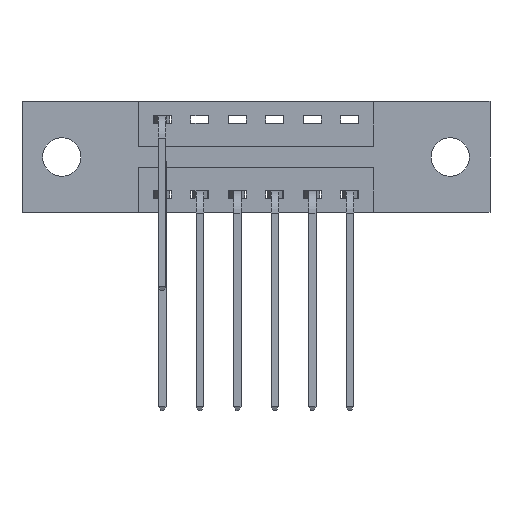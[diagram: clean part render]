
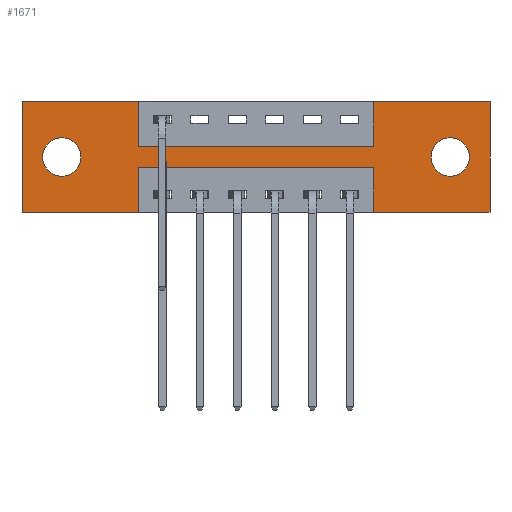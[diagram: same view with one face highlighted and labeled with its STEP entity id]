
A CAD part, front view. The second image highlights one B-rep face of the part: STEP entity #1671.
In plain terms, the highlighted planar face has unit normal (0, -1, 0).
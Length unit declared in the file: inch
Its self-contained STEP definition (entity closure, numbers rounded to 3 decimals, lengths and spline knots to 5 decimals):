
#90 = CARTESIAN_POINT ( 'NONE',  ( 0.3875, 0., -0.15 ) ) ;
#202 = DIRECTION ( 'NONE',  ( -1., 0., 0. ) ) ;
#394 = VERTEX_POINT ( 'NONE', #4883 ) ;
#474 = CARTESIAN_POINT ( 'NONE',  ( 0.3875, 0., 0. ) ) ;
#492 = CARTESIAN_POINT ( 'NONE',  ( 0.3875, 0., 0. ) ) ;
#529 = CARTESIAN_POINT ( 'NONE',  ( 0.3875, 0., -0.37 ) ) ;
#636 = EDGE_LOOP ( 'NONE', ( #1994, #3930 ) ) ;
#640 = DIRECTION ( 'NONE',  ( 0., 0., 1. ) ) ;
#740 = VERTEX_POINT ( 'NONE', #492 ) ;
#747 = DIRECTION ( 'NONE',  ( 0., 1., 0. ) ) ;
#805 = FACE_OUTER_BOUND ( 'NONE', #9752, .T. ) ;
#927 = DIRECTION ( 'NONE',  ( 1., 0., 0. ) ) ;
#945 = VECTOR ( 'NONE', #6337, 39.37008 ) ;
#1133 = DIRECTION ( 'NONE',  ( 0., 1., 0. ) ) ;
#1139 = VERTEX_POINT ( 'NONE', #9438 ) ;
#1234 = VECTOR ( 'NONE', #640, 39.37008 ) ;
#1249 = VERTEX_POINT ( 'NONE', #1520 ) ;
#1357 = FACE_BOUND ( 'NONE', #7469, .T. ) ;
#1470 = EDGE_CURVE ( 'NONE', #5039, #4502, #3247, .T. ) ;
#1492 = LINE ( 'NONE', #8779, #1234 ) ;
#1520 = CARTESIAN_POINT ( 'NONE',  ( 1.1725, 0., -0.15 ) ) ;
#1593 = ORIENTED_EDGE ( 'NONE', *, *, #6274, .F. ) ;
#1630 = AXIS2_PLACEMENT_3D ( 'NONE', #6113, #1133, #6923 ) ;
#1663 = VERTEX_POINT ( 'NONE', #4180 ) ;
#1671 = ADVANCED_FACE ( 'NONE', ( #3384, #1357, #805 ), #9903, .T. ) ;
#1941 = LINE ( 'NONE', #90, #3419 ) ;
#1994 = ORIENTED_EDGE ( 'NONE', *, *, #7190, .T. ) ;
#2124 = VERTEX_POINT ( 'NONE', #6294 ) ;
#2141 = DIRECTION ( 'NONE',  ( 1., 0., 0. ) ) ;
#2580 = LINE ( 'NONE', #8137, #9216 ) ;
#2625 = VECTOR ( 'NONE', #4668, 39.37008 ) ;
#2714 = EDGE_CURVE ( 'NONE', #3999, #8539, #7148, .T. ) ;
#2780 = AXIS2_PLACEMENT_3D ( 'NONE', #9144, #7848, #4446 ) ;
#2950 = CIRCLE ( 'NONE', #5992, 0.064 ) ;
#2985 = ORIENTED_EDGE ( 'NONE', *, *, #6640, .T. ) ;
#3200 = EDGE_CURVE ( 'NONE', #394, #6590, #8996, .T. ) ;
#3211 = ORIENTED_EDGE ( 'NONE', *, *, #8750, .F. ) ;
#3247 = LINE ( 'NONE', #10345, #9323 ) ;
#3329 = CARTESIAN_POINT ( 'NONE',  ( 1.4275, 0., -0.185 ) ) ;
#3384 = FACE_BOUND ( 'NONE', #636, .T. ) ;
#3402 = ORIENTED_EDGE ( 'NONE', *, *, #3988, .F. ) ;
#3419 = VECTOR ( 'NONE', #927, 39.37008 ) ;
#3431 = EDGE_CURVE ( 'NONE', #740, #1663, #4963, .T. ) ;
#3490 = ORIENTED_EDGE ( 'NONE', *, *, #9827, .T. ) ;
#3673 = CARTESIAN_POINT ( 'NONE',  ( 0., 0., 0. ) ) ;
#3804 = ORIENTED_EDGE ( 'NONE', *, *, #5069, .F. ) ;
#3930 = ORIENTED_EDGE ( 'NONE', *, *, #2714, .T. ) ;
#3988 = EDGE_CURVE ( 'NONE', #1663, #1249, #1941, .T. ) ;
#3999 = VERTEX_POINT ( 'NONE', #5901 ) ;
#4078 = CARTESIAN_POINT ( 'NONE',  ( 0., 0., 0. ) ) ;
#4165 = DIRECTION ( 'NONE',  ( 0., 0., -1. ) ) ;
#4180 = CARTESIAN_POINT ( 'NONE',  ( 0.3875, 0., -0.15 ) ) ;
#4211 = DIRECTION ( 'NONE',  ( 0., 0., 1. ) ) ;
#4364 = CIRCLE ( 'NONE', #9843, 0.064 ) ;
#4430 = CARTESIAN_POINT ( 'NONE',  ( 0., 0., -0.37 ) ) ;
#4446 = DIRECTION ( 'NONE',  ( 0., 0., -1. ) ) ;
#4502 = VERTEX_POINT ( 'NONE', #7299 ) ;
#4541 = EDGE_CURVE ( 'NONE', #1249, #7919, #2580, .T. ) ;
#4642 = DIRECTION ( 'NONE',  ( 0., -1., 0. ) ) ;
#4668 = DIRECTION ( 'NONE',  ( -1., 0., 0. ) ) ;
#4714 = DIRECTION ( 'NONE',  ( 0., 0., -1. ) ) ;
#4853 = VECTOR ( 'NONE', #6493, 39.37008 ) ;
#4883 = CARTESIAN_POINT ( 'NONE',  ( 0., 0., -0.37 ) ) ;
#4946 = CARTESIAN_POINT ( 'NONE',  ( 0., 0., -0.37 ) ) ;
#4963 = LINE ( 'NONE', #474, #6814 ) ;
#5039 = VERTEX_POINT ( 'NONE', #7229 ) ;
#5069 = EDGE_CURVE ( 'NONE', #10313, #1139, #1492, .T. ) ;
#5149 = ORIENTED_EDGE ( 'NONE', *, *, #1470, .F. ) ;
#5151 = LINE ( 'NONE', #10004, #7263 ) ;
#5500 = LINE ( 'NONE', #7042, #5964 ) ;
#5536 = ORIENTED_EDGE ( 'NONE', *, *, #8371, .F. ) ;
#5548 = CARTESIAN_POINT ( 'NONE',  ( 0.3875, 0., -0.22 ) ) ;
#5590 = EDGE_CURVE ( 'NONE', #1139, #8738, #9538, .T. ) ;
#5673 = CARTESIAN_POINT ( 'NONE',  ( 0.1325, 0., -0.121 ) ) ;
#5721 = CARTESIAN_POINT ( 'NONE',  ( 1.1725, 0., 0. ) ) ;
#5766 = CARTESIAN_POINT ( 'NONE',  ( 0.1325, 0., -0.185 ) ) ;
#5901 = CARTESIAN_POINT ( 'NONE',  ( 1.4275, 0., -0.249 ) ) ;
#5964 = VECTOR ( 'NONE', #2141, 39.37008 ) ;
#5985 = DIRECTION ( 'NONE',  ( 0., 0., -1. ) ) ;
#5990 = LINE ( 'NONE', #4078, #9882 ) ;
#5992 = AXIS2_PLACEMENT_3D ( 'NONE', #3329, #8870, #4165 ) ;
#6084 = ORIENTED_EDGE ( 'NONE', *, *, #3200, .F. ) ;
#6113 = CARTESIAN_POINT ( 'NONE',  ( 0.1325, 0., -0.185 ) ) ;
#6122 = EDGE_CURVE ( 'NONE', #8738, #7765, #5151, .T. ) ;
#6209 = DIRECTION ( 'NONE',  ( 0., 0., -1. ) ) ;
#6225 = LINE ( 'NONE', #4430, #8057 ) ;
#6274 = EDGE_CURVE ( 'NONE', #7919, #5039, #5990, .T. ) ;
#6278 = VERTEX_POINT ( 'NONE', #5673 ) ;
#6294 = CARTESIAN_POINT ( 'NONE',  ( 0.1325, 0., -0.249 ) ) ;
#6337 = DIRECTION ( 'NONE',  ( -1., 0., 0. ) ) ;
#6464 = DIRECTION ( 'NONE',  ( 1., 0., 0. ) ) ;
#6493 = DIRECTION ( 'NONE',  ( 0., 0., 1. ) ) ;
#6558 = DIRECTION ( 'NONE',  ( 0., 0., 1. ) ) ;
#6590 = VERTEX_POINT ( 'NONE', #3673 ) ;
#6640 = EDGE_CURVE ( 'NONE', #6278, #2124, #6899, .T. ) ;
#6739 = CARTESIAN_POINT ( 'NONE',  ( 0.3875, 0., -0.22 ) ) ;
#6814 = VECTOR ( 'NONE', #4714, 39.37008 ) ;
#6899 = CIRCLE ( 'NONE', #1630, 0.064 ) ;
#6923 = DIRECTION ( 'NONE',  ( 0., 0., 1. ) ) ;
#6925 = ORIENTED_EDGE ( 'NONE', *, *, #6122, .F. ) ;
#7042 = CARTESIAN_POINT ( 'NONE',  ( 0., 0., 0. ) ) ;
#7072 = ORIENTED_EDGE ( 'NONE', *, *, #3431, .F. ) ;
#7148 = CIRCLE ( 'NONE', #2780, 0.064 ) ;
#7190 = EDGE_CURVE ( 'NONE', #8539, #3999, #2950, .T. ) ;
#7229 = CARTESIAN_POINT ( 'NONE',  ( 1.56, 0., 0. ) ) ;
#7263 = VECTOR ( 'NONE', #9251, 39.37008 ) ;
#7299 = CARTESIAN_POINT ( 'NONE',  ( 1.56, 0., -0.37 ) ) ;
#7375 = CARTESIAN_POINT ( 'NONE',  ( 1.4275, 0., -0.121 ) ) ;
#7469 = EDGE_LOOP ( 'NONE', ( #2985, #3490 ) ) ;
#7765 = VERTEX_POINT ( 'NONE', #529 ) ;
#7848 = DIRECTION ( 'NONE',  ( 0., 1., 0. ) ) ;
#7918 = CARTESIAN_POINT ( 'NONE',  ( 1.1725, 0., -0.37 ) ) ;
#7919 = VERTEX_POINT ( 'NONE', #5721 ) ;
#8008 = ORIENTED_EDGE ( 'NONE', *, *, #5590, .F. ) ;
#8057 = VECTOR ( 'NONE', #202, 39.37008 ) ;
#8137 = CARTESIAN_POINT ( 'NONE',  ( 1.1725, 0., 0. ) ) ;
#8308 = ORIENTED_EDGE ( 'NONE', *, *, #4541, .F. ) ;
#8371 = EDGE_CURVE ( 'NONE', #6590, #740, #5500, .T. ) ;
#8482 = AXIS2_PLACEMENT_3D ( 'NONE', #4946, #4642, #6209 ) ;
#8539 = VERTEX_POINT ( 'NONE', #7375 ) ;
#8738 = VERTEX_POINT ( 'NONE', #6739 ) ;
#8750 = EDGE_CURVE ( 'NONE', #7765, #394, #6225, .T. ) ;
#8779 = CARTESIAN_POINT ( 'NONE',  ( 1.1725, 0., -0.37 ) ) ;
#8787 = LINE ( 'NONE', #9335, #2625 ) ;
#8870 = DIRECTION ( 'NONE',  ( 0., 1., 0. ) ) ;
#8961 = CARTESIAN_POINT ( 'NONE',  ( 0., 0., 0. ) ) ;
#8996 = LINE ( 'NONE', #8961, #4853 ) ;
#9144 = CARTESIAN_POINT ( 'NONE',  ( 1.4275, 0., -0.185 ) ) ;
#9216 = VECTOR ( 'NONE', #4211, 39.37008 ) ;
#9227 = ORIENTED_EDGE ( 'NONE', *, *, #10240, .F. ) ;
#9251 = DIRECTION ( 'NONE',  ( 0., 0., -1. ) ) ;
#9323 = VECTOR ( 'NONE', #5985, 39.37008 ) ;
#9335 = CARTESIAN_POINT ( 'NONE',  ( 0., 0., -0.37 ) ) ;
#9438 = CARTESIAN_POINT ( 'NONE',  ( 1.1725, 0., -0.22 ) ) ;
#9538 = LINE ( 'NONE', #5548, #945 ) ;
#9752 = EDGE_LOOP ( 'NONE', ( #6925, #8008, #3804, #9227, #5149, #1593, #8308, #3402, #7072, #5536, #6084, #3211 ) ) ;
#9827 = EDGE_CURVE ( 'NONE', #2124, #6278, #4364, .T. ) ;
#9843 = AXIS2_PLACEMENT_3D ( 'NONE', #5766, #747, #6558 ) ;
#9882 = VECTOR ( 'NONE', #6464, 39.37008 ) ;
#9903 = PLANE ( 'NONE',  #8482 ) ;
#10004 = CARTESIAN_POINT ( 'NONE',  ( 0.3875, 0., -0.37 ) ) ;
#10240 = EDGE_CURVE ( 'NONE', #4502, #10313, #8787, .T. ) ;
#10313 = VERTEX_POINT ( 'NONE', #7918 ) ;
#10345 = CARTESIAN_POINT ( 'NONE',  ( 1.56, 0., 0. ) ) ;
